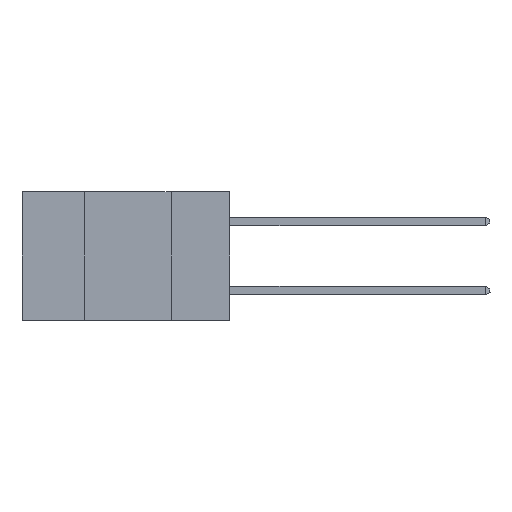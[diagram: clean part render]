
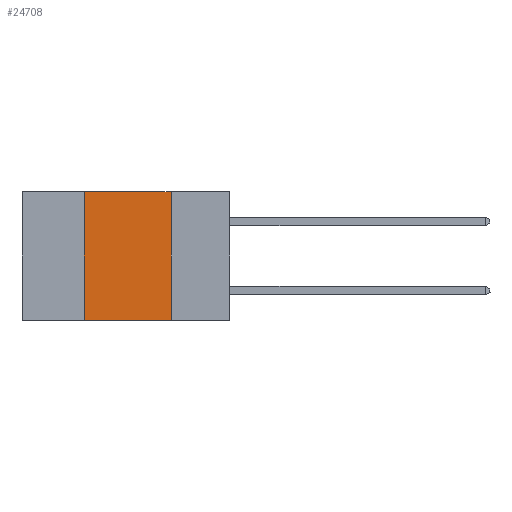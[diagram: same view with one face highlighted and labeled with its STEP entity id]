
A CAD part, left-side view. The second image highlights one B-rep face of the part: STEP entity #24708.
In plain terms, the highlighted planar face has unit normal (-1, 0, 0).
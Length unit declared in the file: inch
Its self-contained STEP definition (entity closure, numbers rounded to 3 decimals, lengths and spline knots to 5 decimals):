
#53 = ORIENTED_EDGE ( 'NONE', *, *, #4788, .T. ) ;
#1738 = ORIENTED_EDGE ( 'NONE', *, *, #5982, .F. ) ;
#2671 = EDGE_CURVE ( 'NONE', #26739, #17993, #9221, .T. ) ;
#2791 = DIRECTION ( 'NONE',  ( 0., 0., -1. ) ) ;
#3958 = CARTESIAN_POINT ( 'NONE',  ( 0., 0.42, -0.37 ) ) ;
#4294 = EDGE_CURVE ( 'NONE', #17993, #13714, #11840, .T. ) ;
#4788 = EDGE_CURVE ( 'NONE', #19480, #13714, #21154, .T. ) ;
#4858 = VECTOR ( 'NONE', #6766, 39.37008 ) ;
#5076 = VECTOR ( 'NONE', #25990, 39.37008 ) ;
#5324 = ORIENTED_EDGE ( 'NONE', *, *, #2671, .F. ) ;
#5415 = CARTESIAN_POINT ( 'NONE',  ( 0., 0.17, 0. ) ) ;
#5982 = EDGE_CURVE ( 'NONE', #19480, #26739, #15880, .T. ) ;
#6679 = CARTESIAN_POINT ( 'NONE',  ( 0., 0.6, 0. ) ) ;
#6766 = DIRECTION ( 'NONE',  ( 0., 0., 1. ) ) ;
#8050 = VECTOR ( 'NONE', #27739, 39.37008 ) ;
#9221 = LINE ( 'NONE', #10517, #5076 ) ;
#10059 = FACE_OUTER_BOUND ( 'NONE', #28015, .T. ) ;
#10517 = CARTESIAN_POINT ( 'NONE',  ( 0., 0.6, 0. ) ) ;
#11840 = LINE ( 'NONE', #5415, #8050 ) ;
#13714 = VERTEX_POINT ( 'NONE', #26642 ) ;
#15880 = LINE ( 'NONE', #19911, #4858 ) ;
#16766 = DIRECTION ( 'NONE',  ( 0., -1., 0. ) ) ;
#17667 = AXIS2_PLACEMENT_3D ( 'NONE', #6679, #22127, #2791 ) ;
#17993 = VERTEX_POINT ( 'NONE', #20308 ) ;
#19480 = VERTEX_POINT ( 'NONE', #3958 ) ;
#19871 = ORIENTED_EDGE ( 'NONE', *, *, #4294, .F. ) ;
#19911 = CARTESIAN_POINT ( 'NONE',  ( 0., 0.42, 0. ) ) ;
#20308 = CARTESIAN_POINT ( 'NONE',  ( 0., 0.17, 0. ) ) ;
#20383 = CARTESIAN_POINT ( 'NONE',  ( 0., 0.6, -0.37 ) ) ;
#20856 = CARTESIAN_POINT ( 'NONE',  ( 0., 0.42, 0. ) ) ;
#21154 = LINE ( 'NONE', #20383, #24611 ) ;
#22127 = DIRECTION ( 'NONE',  ( 1., 0., 0. ) ) ;
#24611 = VECTOR ( 'NONE', #16766, 39.37008 ) ;
#24708 = ADVANCED_FACE ( 'NONE', ( #10059 ), #26849, .F. ) ;
#25990 = DIRECTION ( 'NONE',  ( 0., -1., 0. ) ) ;
#26642 = CARTESIAN_POINT ( 'NONE',  ( 0., 0.17, -0.37 ) ) ;
#26739 = VERTEX_POINT ( 'NONE', #20856 ) ;
#26849 = PLANE ( 'NONE',  #17667 ) ;
#27739 = DIRECTION ( 'NONE',  ( 0., 0., -1. ) ) ;
#28015 = EDGE_LOOP ( 'NONE', ( #19871, #5324, #1738, #53 ) ) ;
